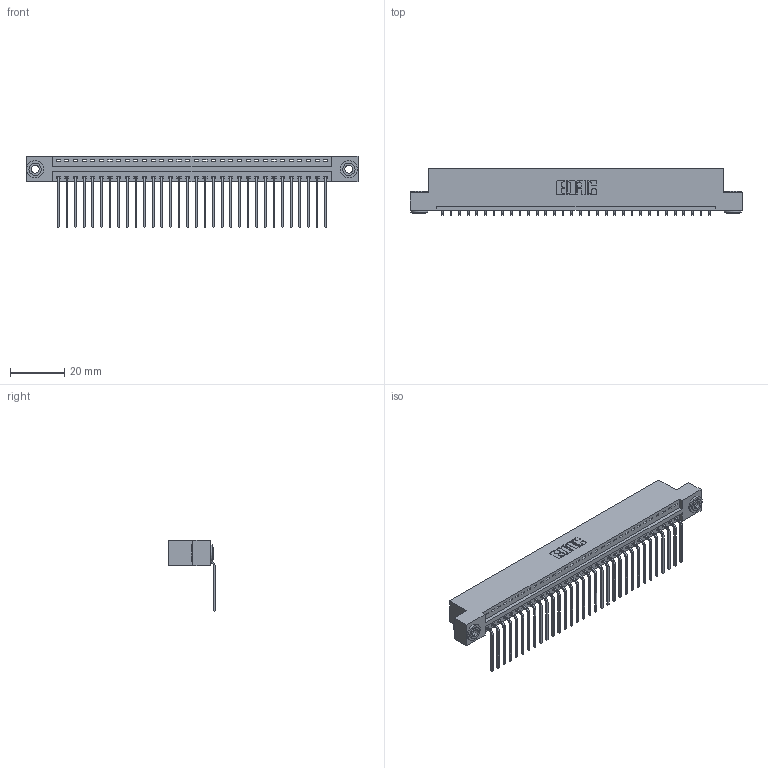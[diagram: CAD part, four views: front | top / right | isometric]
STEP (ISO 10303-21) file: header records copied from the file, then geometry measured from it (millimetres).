
FILE_DESCRIPTION (( 'STEP AP203' ), '1' );
FILE_NAME ('346-032-559-103.STEP', '2022-05-06T18:56:15', ( '' ), ( '' ), 'SwSTEP 2.0', 'SolidWorks 2020', '' );
FILE_SCHEMA (( 'CONFIG_CONTROL_DESIGN' ));
Length unit declared in the file: inch
Products named in the file (4): 345-292-001_558 559 Tail - 1; 346-032-559-103; 345-250-002_345-250-002-102; 346 Part_Flush Mounting Lugs - 0.156 Dia-TH
Assembly tree (35 placements, depth 2):
  346-032-559-103
    346 Part_Flush Mounting Lugs - 0.156 Dia-TH
    345-292-001_558 559 Tail - 1  x32
    345-250-002_345-250-002-102  x2
Bounding box: 122.17 x 17.08 x 26.16 mm (x, y, z)
Volume: 11733.8 mm3; surface area: 15445.3 mm2
Topology: 35 solids, 35 shells, 2094 faces, 6265 edges, 4130 vertices
Faces by surface type: plane 1444, cylinder 642, cone 8
Entity records: 22356 total; most frequent: CARTESIAN_POINT 3817, ORIENTED_EDGE 3774, DIRECTION 3409, EDGE_CURVE 1887, LINE 1603, VECTOR 1603, VERTEX_POINT 1254, AXIS2_PLACEMENT_3D 903
